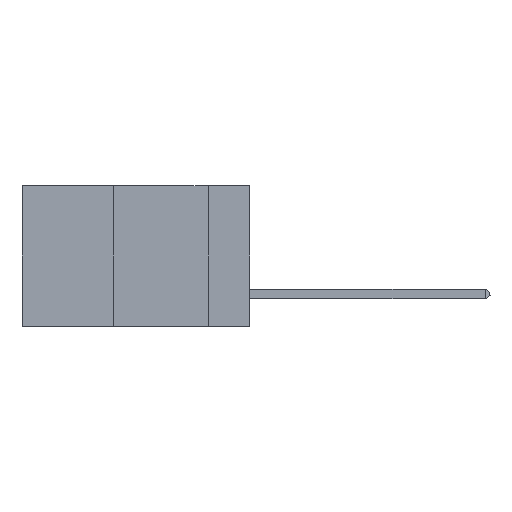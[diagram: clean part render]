
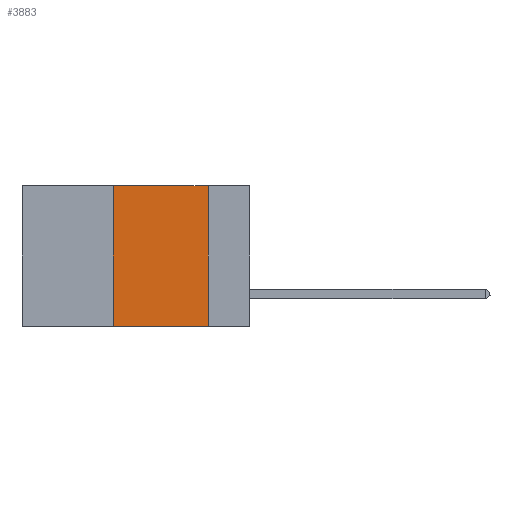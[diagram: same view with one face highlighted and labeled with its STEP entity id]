
A CAD part, left-side view. The second image highlights one B-rep face of the part: STEP entity #3883.
In plain terms, the highlighted planar face has unit normal (-1, 0, 0).
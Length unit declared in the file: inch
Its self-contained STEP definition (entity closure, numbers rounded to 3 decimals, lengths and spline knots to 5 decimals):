
#617 = ORIENTED_EDGE ( 'NONE', *, *, #15985, .F. ) ;
#2525 = CARTESIAN_POINT ( 'NONE',  ( 0., 0.11, 0. ) ) ;
#3143 = CARTESIAN_POINT ( 'NONE',  ( 0., 0.36, 0. ) ) ;
#3883 = ADVANCED_FACE ( 'NONE', ( #21517 ), #23491, .F. ) ;
#4088 = EDGE_LOOP ( 'NONE', ( #617, #11841, #22338, #25386 ) ) ;
#4458 = DIRECTION ( 'NONE',  ( 1., 0., 0. ) ) ;
#4741 = VECTOR ( 'NONE', #5865, 39.37008 ) ;
#4829 = CARTESIAN_POINT ( 'NONE',  ( 0., 0.6, 0. ) ) ;
#5655 = CARTESIAN_POINT ( 'NONE',  ( 0., 0.36, -0.37 ) ) ;
#5865 = DIRECTION ( 'NONE',  ( 0., 0., 1. ) ) ;
#6286 = LINE ( 'NONE', #7373, #26442 ) ;
#7373 = CARTESIAN_POINT ( 'NONE',  ( 0., 0.11, 0. ) ) ;
#7861 = LINE ( 'NONE', #17465, #14164 ) ;
#8631 = VERTEX_POINT ( 'NONE', #5655 ) ;
#10129 = LINE ( 'NONE', #20476, #4741 ) ;
#10378 = CARTESIAN_POINT ( 'NONE',  ( 0., 0.6, -0.37 ) ) ;
#10904 = EDGE_CURVE ( 'NONE', #23715, #15316, #7861, .T. ) ;
#11841 = ORIENTED_EDGE ( 'NONE', *, *, #10904, .F. ) ;
#14164 = VECTOR ( 'NONE', #20372, 39.37008 ) ;
#15316 = VERTEX_POINT ( 'NONE', #2525 ) ;
#15985 = EDGE_CURVE ( 'NONE', #15316, #26485, #6286, .T. ) ;
#17465 = CARTESIAN_POINT ( 'NONE',  ( 0., 0.6, 0. ) ) ;
#17485 = CARTESIAN_POINT ( 'NONE',  ( 0., 0.11, -0.37 ) ) ;
#17691 = DIRECTION ( 'NONE',  ( 0., 0., -1. ) ) ;
#18844 = DIRECTION ( 'NONE',  ( 0., -1., 0. ) ) ;
#19181 = AXIS2_PLACEMENT_3D ( 'NONE', #4829, #4458, #17691 ) ;
#19819 = DIRECTION ( 'NONE',  ( 0., 0., -1. ) ) ;
#20372 = DIRECTION ( 'NONE',  ( 0., -1., 0. ) ) ;
#20476 = CARTESIAN_POINT ( 'NONE',  ( 0., 0.36, 0. ) ) ;
#21517 = FACE_OUTER_BOUND ( 'NONE', #4088, .T. ) ;
#21651 = VECTOR ( 'NONE', #18844, 39.37008 ) ;
#22338 = ORIENTED_EDGE ( 'NONE', *, *, #23825, .F. ) ;
#23295 = EDGE_CURVE ( 'NONE', #8631, #26485, #27238, .T. ) ;
#23491 = PLANE ( 'NONE',  #19181 ) ;
#23715 = VERTEX_POINT ( 'NONE', #3143 ) ;
#23825 = EDGE_CURVE ( 'NONE', #8631, #23715, #10129, .T. ) ;
#25386 = ORIENTED_EDGE ( 'NONE', *, *, #23295, .T. ) ;
#26442 = VECTOR ( 'NONE', #19819, 39.37008 ) ;
#26485 = VERTEX_POINT ( 'NONE', #17485 ) ;
#27238 = LINE ( 'NONE', #10378, #21651 ) ;
